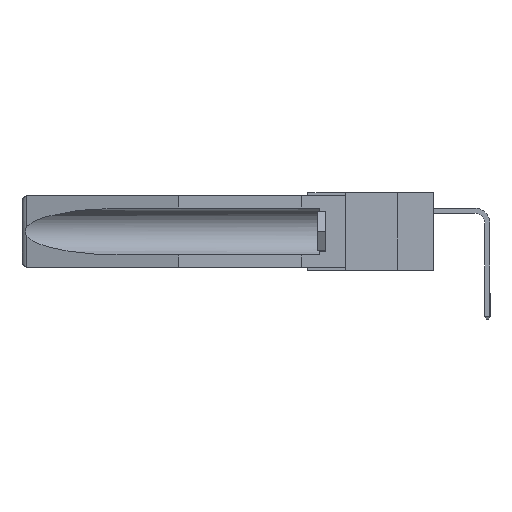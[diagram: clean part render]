
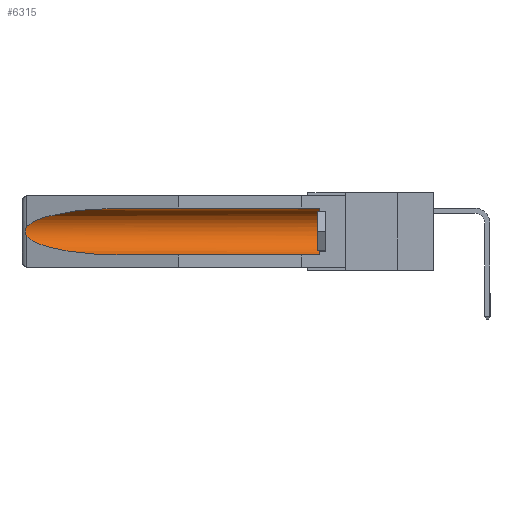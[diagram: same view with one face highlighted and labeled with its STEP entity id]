
A CAD part, left-side view. The second image highlights one B-rep face of the part: STEP entity #6315.
In plain terms, the highlighted cylindrical face has radius 2.857 mm (diameter 5.715 mm), a partial arc.
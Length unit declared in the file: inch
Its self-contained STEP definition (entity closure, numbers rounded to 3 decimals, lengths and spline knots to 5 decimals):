
#780 = ORIENTED_EDGE ( 'NONE', *, *, #16224, .T. ) ;
#880 = CARTESIAN_POINT ( 'NONE',  ( 0.155, 1.07973, -0.059 ) ) ;
#1066 = CARTESIAN_POINT ( 'NONE',  ( 0.155, 1.07973, -0.284 ) ) ;
#1520 = VERTEX_POINT ( 'NONE', #1066 ) ;
#1564 = CARTESIAN_POINT ( 'NONE',  ( 0.25451, 1.48313, -0.09465 ) ) ;
#1762 = CARTESIAN_POINT ( 'NONE',  ( 0.26655, 1.53094, -0.18657 ) ) ;
#1779 = VERTEX_POINT ( 'NONE', #13668 ) ;
#1943 = AXIS2_PLACEMENT_3D ( 'NONE', #17991, #8018, #5898 ) ;
#2272 = CARTESIAN_POINT ( 'NONE',  ( 0.155, -0.30754, -0.284 ) ) ;
#2277 = VERTEX_POINT ( 'NONE', #14286 ) ;
#2288 = CARTESIAN_POINT ( 'NONE',  ( 0.26597, 1.5296, -0.19026 ) ) ;
#2452 = VERTEX_POINT ( 'NONE', #10161 ) ;
#4787 = CARTESIAN_POINT ( 'NONE',  ( 0.155, -0.30754, -0.059 ) ) ;
#5436 = ORIENTED_EDGE ( 'NONE', *, *, #17043, .F. ) ;
#5898 = DIRECTION ( 'NONE',  ( 0., 0., 1. ) ) ;
#5955 = CARTESIAN_POINT ( 'NONE',  ( 0.155, 1.07973, -0.059 ) ) ;
#6315 = ADVANCED_FACE ( 'NONE', ( #6828 ), #24113, .F. ) ;
#6420 = VECTOR ( 'NONE', #19112, 39.37008 ) ;
#6828 = FACE_OUTER_BOUND ( 'NONE', #15735, .T. ) ;
#7105 = VERTEX_POINT ( 'NONE', #18573 ) ;
#8014 = CARTESIAN_POINT ( 'NONE',  ( 0.26597, 1.52961, -0.15275 ) ) ;
#8018 = DIRECTION ( 'NONE',  ( 0., 1., 0. ) ) ;
#8668 = LINE ( 'NONE', #2272, #16730 ) ;
#9328 = VERTEX_POINT ( 'NONE', #880 ) ;
#9385 = DIRECTION ( 'NONE',  ( 0., -1., 0. ) ) ;
#9801 = CARTESIAN_POINT ( 'NONE',  ( 0.2673, 1.53269, -0.17917 ) ) ;
#10154 = DIRECTION ( 'NONE',  ( 0., 1., 0. ) ) ;
#10161 = CARTESIAN_POINT ( 'NONE',  ( 0.26537, 1.52718, -0.14972 ) ) ;
#10625 = CARTESIAN_POINT ( 'NONE',  ( 0.26537, 1.52718, -0.19328 ) ) ;
#10985 =( BOUNDED_CURVE ( )  B_SPLINE_CURVE ( 3, ( #5955, #14018, #1564, #26427 ),
 .UNSPECIFIED., .F., .F. ) 
 B_SPLINE_CURVE_WITH_KNOTS ( ( 4, 4 ),
 ( 4.71239, 6.08839 ),
 .UNSPECIFIED. ) 
 CURVE ( )  GEOMETRIC_REPRESENTATION_ITEM ( )  RATIONAL_B_SPLINE_CURVE ( ( 1., 0.848, 0.848, 1. ) ) 
 REPRESENTATION_ITEM ( '' )  );
#11193 = CARTESIAN_POINT ( 'NONE',  ( 0.155, 1.07973, -0.284 ) ) ;
#11688 = EDGE_CURVE ( 'NONE', #9328, #2452, #10985, .T. ) ;
#12025 = ORIENTED_EDGE ( 'NONE', *, *, #23861, .T. ) ;
#12245 = CARTESIAN_POINT ( 'NONE',  ( 0.2675, 1.53308, -0.16763 ) ) ;
#12854 = CIRCLE ( 'NONE', #18755, 0.1125 ) ;
#13668 = CARTESIAN_POINT ( 'NONE',  ( 0.26537, 1.52718, -0.19328 ) ) ;
#13873 = CARTESIAN_POINT ( 'NONE',  ( 0.2675, 1.53308, -0.17534 ) ) ;
#14018 = CARTESIAN_POINT ( 'NONE',  ( 0.21114, 1.30732, -0.059 ) ) ;
#14286 = CARTESIAN_POINT ( 'NONE',  ( 0.155, 0.126, -0.284 ) ) ;
#14472 = LINE ( 'NONE', #4787, #6420 ) ;
#15433 = DIRECTION ( 'NONE',  ( 0., 0., 1. ) ) ;
#15735 = EDGE_LOOP ( 'NONE', ( #16270, #780, #17593, #5436, #12025, #23064 ) ) ;
#16224 = EDGE_CURVE ( 'NONE', #2452, #1779, #20119, .T. ) ;
#16270 = ORIENTED_EDGE ( 'NONE', *, *, #11688, .T. ) ;
#16730 = VECTOR ( 'NONE', #10154, 39.37008 ) ;
#16852 =( BOUNDED_CURVE ( )  B_SPLINE_CURVE ( 3, ( #23330, #21096, #25466, #11193 ),
 .UNSPECIFIED., .F., .F. ) 
 B_SPLINE_CURVE_WITH_KNOTS ( ( 4, 4 ),
 ( 0.1948, 1.5708 ),
 .UNSPECIFIED. ) 
 CURVE ( )  GEOMETRIC_REPRESENTATION_ITEM ( )  RATIONAL_B_SPLINE_CURVE ( ( 1., 0.848, 0.848, 1. ) ) 
 REPRESENTATION_ITEM ( '' )  );
#17043 = EDGE_CURVE ( 'NONE', #2277, #1520, #8668, .T. ) ;
#17470 = CARTESIAN_POINT ( 'NONE',  ( 0.155, 0.126, -0.1715 ) ) ;
#17593 = ORIENTED_EDGE ( 'NONE', *, *, #26236, .T. ) ;
#17991 = CARTESIAN_POINT ( 'NONE',  ( 0.155, -0.30754, -0.1715 ) ) ;
#18079 = EDGE_CURVE ( 'NONE', #7105, #9328, #14472, .T. ) ;
#18162 = CARTESIAN_POINT ( 'NONE',  ( 0.2673, 1.5327, -0.16383 ) ) ;
#18573 = CARTESIAN_POINT ( 'NONE',  ( 0.155, 0.126, -0.059 ) ) ;
#18755 = AXIS2_PLACEMENT_3D ( 'NONE', #17470, #9385, #15433 ) ;
#19112 = DIRECTION ( 'NONE',  ( 0., 1., 0. ) ) ;
#20119 = B_SPLINE_CURVE_WITH_KNOTS ( 'NONE', 3,
 ( #24217, #8014, #20357, #18162, #12245, #13873, #9801, #1762, #2288, #10625 ),
 .UNSPECIFIED., .F., .F.,
 ( 4, 2, 2, 2, 4 ),
 ( 0., 0.00029, 0.00058, 0.00087, 0.00117 ),
 .UNSPECIFIED. ) ;
#20357 = CARTESIAN_POINT ( 'NONE',  ( 0.26654, 1.53092, -0.15636 ) ) ;
#21096 = CARTESIAN_POINT ( 'NONE',  ( 0.25451, 1.48313, -0.24835 ) ) ;
#23064 = ORIENTED_EDGE ( 'NONE', *, *, #18079, .T. ) ;
#23330 = CARTESIAN_POINT ( 'NONE',  ( 0.26537, 1.52718, -0.19328 ) ) ;
#23861 = EDGE_CURVE ( 'NONE', #2277, #7105, #12854, .T. ) ;
#24113 = CYLINDRICAL_SURFACE ( 'NONE', #1943, 0.1125 ) ;
#24217 = CARTESIAN_POINT ( 'NONE',  ( 0.26537, 1.52718, -0.14972 ) ) ;
#25466 = CARTESIAN_POINT ( 'NONE',  ( 0.21114, 1.30732, -0.284 ) ) ;
#26236 = EDGE_CURVE ( 'NONE', #1779, #1520, #16852, .T. ) ;
#26427 = CARTESIAN_POINT ( 'NONE',  ( 0.26537, 1.52718, -0.14972 ) ) ;
